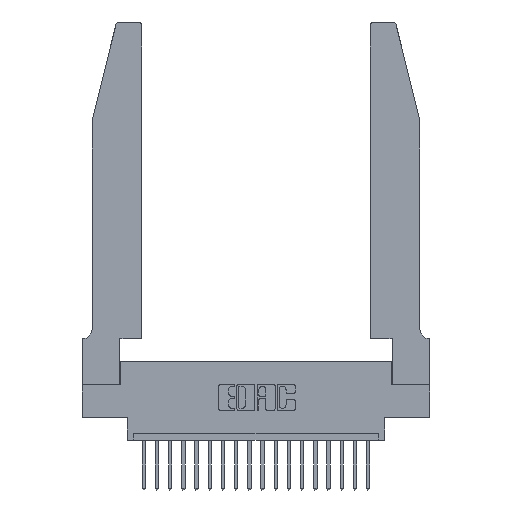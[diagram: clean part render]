
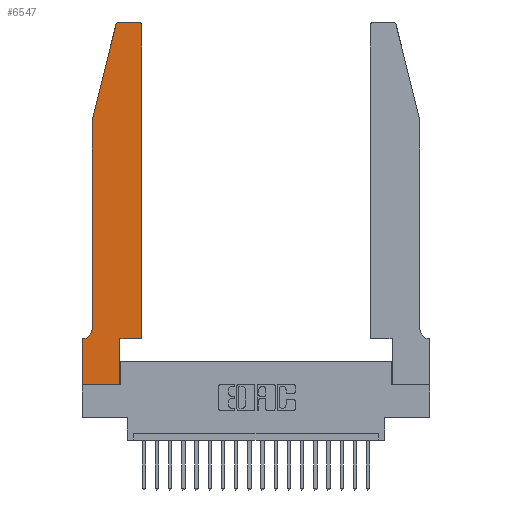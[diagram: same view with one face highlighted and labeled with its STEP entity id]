
A CAD part, top view. The second image highlights one B-rep face of the part: STEP entity #6547.
In plain terms, the highlighted planar face has unit normal (0, 0, 1).
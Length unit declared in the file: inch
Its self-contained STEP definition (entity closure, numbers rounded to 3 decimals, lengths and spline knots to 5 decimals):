
#81 = AXIS2_PLACEMENT_3D ( 'NONE', #3851, #2413, #10717 ) ;
#533 = VERTEX_POINT ( 'NONE', #18240 ) ;
#571 = DIRECTION ( 'NONE',  ( 0., -1., 0. ) ) ;
#591 = ORIENTED_EDGE ( 'NONE', *, *, #11363, .T. ) ;
#1648 = EDGE_CURVE ( 'NONE', #14521, #533, #10219, .T. ) ;
#2009 = DIRECTION ( 'NONE',  ( 1., 0., 0. ) ) ;
#2413 = DIRECTION ( 'NONE',  ( 0., 0., 1. ) ) ;
#2419 = LINE ( 'NONE', #15010, #14393 ) ;
#2512 = DIRECTION ( 'NONE',  ( -1., 0., 0. ) ) ;
#2980 = CARTESIAN_POINT ( 'NONE',  ( 0.4205, 2.72, 0.37 ) ) ;
#3662 = ORIENTED_EDGE ( 'NONE', *, *, #21329, .T. ) ;
#3851 = CARTESIAN_POINT ( 'NONE',  ( 0.284, 2.72, 0.37 ) ) ;
#3889 = EDGE_CURVE ( 'NONE', #5921, #16231, #20309, .T. ) ;
#4429 = ORIENTED_EDGE ( 'NONE', *, *, #21134, .T. ) ;
#4543 = ORIENTED_EDGE ( 'NONE', *, *, #19640, .T. ) ;
#4846 = EDGE_CURVE ( 'NONE', #16444, #11232, #6959, .T. ) ;
#4947 = ORIENTED_EDGE ( 'NONE', *, *, #16785, .T. ) ;
#4983 = EDGE_CURVE ( 'NONE', #16772, #9502, #18171, .T. ) ;
#5436 = VERTEX_POINT ( 'NONE', #12873 ) ;
#5921 = VERTEX_POINT ( 'NONE', #11944 ) ;
#5962 = VERTEX_POINT ( 'NONE', #6331 ) ;
#5998 = AXIS2_PLACEMENT_3D ( 'NONE', #12963, #16267, #13191 ) ;
#6135 = LINE ( 'NONE', #17629, #9011 ) ;
#6324 = DIRECTION ( 'NONE',  ( 0., 0., 1. ) ) ;
#6331 = CARTESIAN_POINT ( 'NONE',  ( 0.25487, 2.72718, 0.37 ) ) ;
#6467 = ORIENTED_EDGE ( 'NONE', *, *, #4846, .T. ) ;
#6547 = ADVANCED_FACE ( 'NONE', ( #13543 ), #7836, .T. ) ;
#6661 = ORIENTED_EDGE ( 'NONE', *, *, #4983, .T. ) ;
#6866 = CARTESIAN_POINT ( 'NONE',  ( 0.2865, 0.35, 0.37 ) ) ;
#6959 = LINE ( 'NONE', #17412, #15573 ) ;
#7020 = CARTESIAN_POINT ( 'NONE',  ( 0., 0., 0.37 ) ) ;
#7066 = LINE ( 'NONE', #15462, #17015 ) ;
#7239 = VERTEX_POINT ( 'NONE', #6866 ) ;
#7836 = PLANE ( 'NONE',  #15021 ) ;
#9011 = VECTOR ( 'NONE', #21311, 39.37008 ) ;
#9182 = CIRCLE ( 'NONE', #20281, 0.03 ) ;
#9297 = EDGE_CURVE ( 'NONE', #533, #7239, #6135, .T. ) ;
#9307 = EDGE_CURVE ( 'NONE', #14820, #5436, #17399, .T. ) ;
#9460 = ORIENTED_EDGE ( 'NONE', *, *, #9307, .T. ) ;
#9498 = CARTESIAN_POINT ( 'NONE',  ( 0.4205, 2.75, 0.37 ) ) ;
#9502 = VERTEX_POINT ( 'NONE', #16220 ) ;
#9738 = EDGE_LOOP ( 'NONE', ( #9460, #4543, #3662, #6467, #4429, #6661, #12126, #10231, #10707, #4947, #17140, #591 ) ) ;
#10219 = LINE ( 'NONE', #7020, #10497 ) ;
#10231 = ORIENTED_EDGE ( 'NONE', *, *, #1648, .T. ) ;
#10497 = VECTOR ( 'NONE', #12359, 39.37008 ) ;
#10577 = VECTOR ( 'NONE', #13171, 39.37008 ) ;
#10707 = ORIENTED_EDGE ( 'NONE', *, *, #9297, .T. ) ;
#10717 = DIRECTION ( 'NONE',  ( 1., 0., 0. ) ) ;
#11187 = VECTOR ( 'NONE', #12724, 39.37008 ) ;
#11232 = VERTEX_POINT ( 'NONE', #18765 ) ;
#11363 = EDGE_CURVE ( 'NONE', #16231, #14820, #9182, .T. ) ;
#11448 = LINE ( 'NONE', #18698, #13526 ) ;
#11944 = CARTESIAN_POINT ( 'NONE',  ( 0.4505, 0.35, 0.37 ) ) ;
#12030 = EDGE_CURVE ( 'NONE', #9502, #14521, #7066, .T. ) ;
#12126 = ORIENTED_EDGE ( 'NONE', *, *, #12030, .T. ) ;
#12359 = DIRECTION ( 'NONE',  ( 1., 0., 0. ) ) ;
#12664 = CARTESIAN_POINT ( 'NONE',  ( 0.4505, 0.35, 0.37 ) ) ;
#12710 = CARTESIAN_POINT ( 'NONE',  ( 0., 0.35, 0.37 ) ) ;
#12724 = DIRECTION ( 'NONE',  ( 0., 1., 0. ) ) ;
#12829 = CIRCLE ( 'NONE', #5998, 0.07 ) ;
#12873 = CARTESIAN_POINT ( 'NONE',  ( 0.284, 2.75, 0.37 ) ) ;
#12963 = CARTESIAN_POINT ( 'NONE',  ( 0.0055, 0.42, 0.37 ) ) ;
#13171 = DIRECTION ( 'NONE',  ( -1., 0., 0. ) ) ;
#13191 = DIRECTION ( 'NONE',  ( -1., 0., 0. ) ) ;
#13526 = VECTOR ( 'NONE', #2009, 39.37008 ) ;
#13543 = FACE_OUTER_BOUND ( 'NONE', #9738, .T. ) ;
#13714 = VECTOR ( 'NONE', #2512, 39.37008 ) ;
#14393 = VECTOR ( 'NONE', #18305, 39.37008 ) ;
#14521 = VERTEX_POINT ( 'NONE', #20746 ) ;
#14820 = VERTEX_POINT ( 'NONE', #9498 ) ;
#15010 = CARTESIAN_POINT ( 'NONE',  ( 0.0755, 2., 0.37 ) ) ;
#15021 = AXIS2_PLACEMENT_3D ( 'NONE', #12710, #16087, #19440 ) ;
#15462 = CARTESIAN_POINT ( 'NONE',  ( 0., 0., 0.37 ) ) ;
#15573 = VECTOR ( 'NONE', #20436, 39.37008 ) ;
#16087 = DIRECTION ( 'NONE',  ( 0., 0., 1. ) ) ;
#16220 = CARTESIAN_POINT ( 'NONE',  ( 0., 0.35, 0.37 ) ) ;
#16231 = VERTEX_POINT ( 'NONE', #17510 ) ;
#16267 = DIRECTION ( 'NONE',  ( 0., 0., -1. ) ) ;
#16317 = CIRCLE ( 'NONE', #81, 0.03 ) ;
#16444 = VERTEX_POINT ( 'NONE', #19976 ) ;
#16772 = VERTEX_POINT ( 'NONE', #18627 ) ;
#16785 = EDGE_CURVE ( 'NONE', #7239, #5921, #11448, .T. ) ;
#17015 = VECTOR ( 'NONE', #571, 39.37008 ) ;
#17140 = ORIENTED_EDGE ( 'NONE', *, *, #3889, .T. ) ;
#17399 = LINE ( 'NONE', #20822, #10577 ) ;
#17412 = CARTESIAN_POINT ( 'NONE',  ( 0.0755, 2., 0.37 ) ) ;
#17510 = CARTESIAN_POINT ( 'NONE',  ( 0.4505, 2.72, 0.37 ) ) ;
#17629 = CARTESIAN_POINT ( 'NONE',  ( 0.2865, 0.35, 0.37 ) ) ;
#18002 = DIRECTION ( 'NONE',  ( 1., 0., 0. ) ) ;
#18171 = LINE ( 'NONE', #20816, #13714 ) ;
#18240 = CARTESIAN_POINT ( 'NONE',  ( 0.2865, 0., 0.37 ) ) ;
#18305 = DIRECTION ( 'NONE',  ( -0.239, -0.971, 0. ) ) ;
#18627 = CARTESIAN_POINT ( 'NONE',  ( 0.0055, 0.35, 0.37 ) ) ;
#18698 = CARTESIAN_POINT ( 'NONE',  ( 0.4505, 0.35, 0.37 ) ) ;
#18765 = CARTESIAN_POINT ( 'NONE',  ( 0.0755, 0.42, 0.37 ) ) ;
#19440 = DIRECTION ( 'NONE',  ( 1., 0., 0. ) ) ;
#19640 = EDGE_CURVE ( 'NONE', #5436, #5962, #16317, .T. ) ;
#19976 = CARTESIAN_POINT ( 'NONE',  ( 0.0755, 2., 0.37 ) ) ;
#20281 = AXIS2_PLACEMENT_3D ( 'NONE', #2980, #6324, #18002 ) ;
#20309 = LINE ( 'NONE', #12664, #11187 ) ;
#20436 = DIRECTION ( 'NONE',  ( 0., -1., 0. ) ) ;
#20746 = CARTESIAN_POINT ( 'NONE',  ( 0., 0., 0.37 ) ) ;
#20816 = CARTESIAN_POINT ( 'NONE',  ( 0.0755, 0.35, 0.37 ) ) ;
#20822 = CARTESIAN_POINT ( 'NONE',  ( 0.2605, 2.75, 0.37 ) ) ;
#21134 = EDGE_CURVE ( 'NONE', #11232, #16772, #12829, .T. ) ;
#21311 = DIRECTION ( 'NONE',  ( 0., 1., 0. ) ) ;
#21329 = EDGE_CURVE ( 'NONE', #5962, #16444, #2419, .T. ) ;
